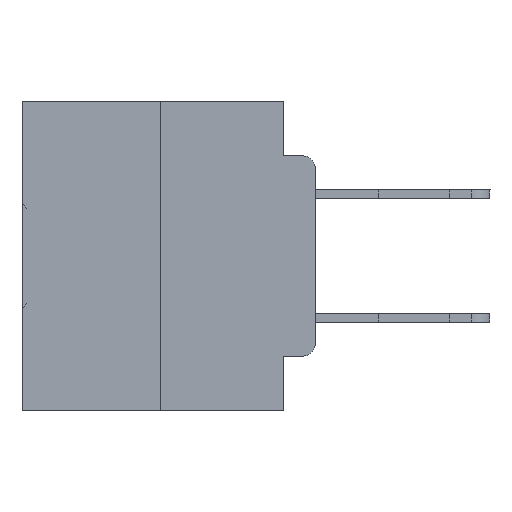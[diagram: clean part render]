
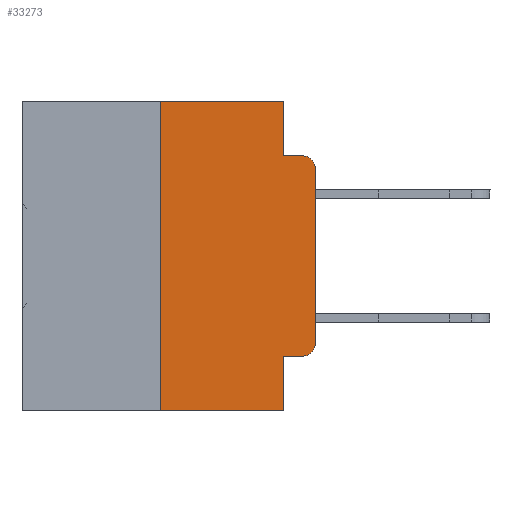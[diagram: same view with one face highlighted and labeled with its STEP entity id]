
A CAD part, left-side view. The second image highlights one B-rep face of the part: STEP entity #33273.
In plain terms, the highlighted planar face has unit normal (-1, 0, 0).
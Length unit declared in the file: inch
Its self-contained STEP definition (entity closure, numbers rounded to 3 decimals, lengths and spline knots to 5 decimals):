
#84 = ORIENTED_EDGE ( 'NONE', *, *, #518, .T. ) ;
#271 = VERTEX_POINT ( 'NONE', #23094 ) ;
#518 = EDGE_CURVE ( 'NONE', #32919, #30354, #25234, .T. ) ;
#638 = CARTESIAN_POINT ( 'NONE',  ( 0., 0.473, -0.5 ) ) ;
#728 = LINE ( 'NONE', #638, #30919 ) ;
#1122 = CARTESIAN_POINT ( 'NONE',  ( 0., 0.051, 0. ) ) ;
#1211 = DIRECTION ( 'NONE',  ( 0., 0., -1. ) ) ;
#1807 = CARTESIAN_POINT ( 'NONE',  ( 0., 0.02, -0.1085 ) ) ;
#1998 = VECTOR ( 'NONE', #28278, 39.37008 ) ;
#2001 = VECTOR ( 'NONE', #23280, 39.37008 ) ;
#2674 = CARTESIAN_POINT ( 'NONE',  ( 0., 0.02, -0.0885 ) ) ;
#3699 = DIRECTION ( 'NONE',  ( 0., -1., 0. ) ) ;
#4699 = CARTESIAN_POINT ( 'NONE',  ( 0., 0.051, -0.0885 ) ) ;
#4810 = CARTESIAN_POINT ( 'NONE',  ( 0., 0.25, 0. ) ) ;
#4901 = FACE_OUTER_BOUND ( 'NONE', #22420, .T. ) ;
#5131 = VERTEX_POINT ( 'NONE', #29912 ) ;
#6466 = LINE ( 'NONE', #28533, #19303 ) ;
#6854 = EDGE_CURVE ( 'NONE', #20907, #25895, #728, .T. ) ;
#7551 = DIRECTION ( 'NONE',  ( -1., 0., 0. ) ) ;
#7661 = ORIENTED_EDGE ( 'NONE', *, *, #16852, .F. ) ;
#8098 = CARTESIAN_POINT ( 'NONE',  ( 0., 0., -0.3915 ) ) ;
#8816 = ORIENTED_EDGE ( 'NONE', *, *, #26133, .T. ) ;
#9095 = CARTESIAN_POINT ( 'NONE',  ( 0., 0.051, -0.4115 ) ) ;
#9280 = ORIENTED_EDGE ( 'NONE', *, *, #27618, .T. ) ;
#10462 = DIRECTION ( 'NONE',  ( 0., 0., -1. ) ) ;
#10625 = ORIENTED_EDGE ( 'NONE', *, *, #31411, .F. ) ;
#11321 = AXIS2_PLACEMENT_3D ( 'NONE', #20862, #7551, #10462 ) ;
#11738 = PLANE ( 'NONE',  #13190 ) ;
#11862 = DIRECTION ( 'NONE',  ( 0., 0., -1. ) ) ;
#12455 = LINE ( 'NONE', #14296, #20310 ) ;
#12686 = DIRECTION ( 'NONE',  ( 0., 0., -1. ) ) ;
#12871 = CARTESIAN_POINT ( 'NONE',  ( 0., 0., -0.1085 ) ) ;
#13122 = CARTESIAN_POINT ( 'NONE',  ( 0., 0.02, -0.4115 ) ) ;
#13190 = AXIS2_PLACEMENT_3D ( 'NONE', #17036, #22673, #1211 ) ;
#14063 = VERTEX_POINT ( 'NONE', #9095 ) ;
#14075 = EDGE_CURVE ( 'NONE', #25152, #5131, #18558, .T. ) ;
#14296 = CARTESIAN_POINT ( 'NONE',  ( 0., 0., 0. ) ) ;
#14378 = LINE ( 'NONE', #1122, #1998 ) ;
#14417 = CARTESIAN_POINT ( 'NONE',  ( 0., 0.473, 0. ) ) ;
#15335 = DIRECTION ( 'NONE',  ( 0., -1., 0. ) ) ;
#15641 = LINE ( 'NONE', #4810, #2001 ) ;
#16852 = EDGE_CURVE ( 'NONE', #20907, #25152, #15641, .T. ) ;
#16993 = ORIENTED_EDGE ( 'NONE', *, *, #14075, .F. ) ;
#17036 = CARTESIAN_POINT ( 'NONE',  ( 0., 0.473, 0. ) ) ;
#17296 = LINE ( 'NONE', #31214, #33454 ) ;
#17738 = AXIS2_PLACEMENT_3D ( 'NONE', #1807, #25504, #11862 ) ;
#18155 = EDGE_CURVE ( 'NONE', #14063, #25895, #6466, .T. ) ;
#18315 = DIRECTION ( 'NONE',  ( 0., -1., 0. ) ) ;
#18558 = LINE ( 'NONE', #14417, #33884 ) ;
#18749 = VERTEX_POINT ( 'NONE', #12871 ) ;
#18763 = CARTESIAN_POINT ( 'NONE',  ( 0., 0.25, 0. ) ) ;
#19303 = VECTOR ( 'NONE', #12686, 39.37008 ) ;
#20310 = VECTOR ( 'NONE', #30365, 39.37008 ) ;
#20862 = CARTESIAN_POINT ( 'NONE',  ( 0., 0.02, -0.3915 ) ) ;
#20907 = VERTEX_POINT ( 'NONE', #31538 ) ;
#22420 = EDGE_LOOP ( 'NONE', ( #8816, #33127, #10625, #22764, #16993, #7661, #24907, #33548, #9280, #84 ) ) ;
#22673 = DIRECTION ( 'NONE',  ( 1., 0., 0. ) ) ;
#22764 = ORIENTED_EDGE ( 'NONE', *, *, #28086, .F. ) ;
#23094 = CARTESIAN_POINT ( 'NONE',  ( 0., 0.051, -0.0885 ) ) ;
#23222 = LINE ( 'NONE', #4699, #32362 ) ;
#23280 = DIRECTION ( 'NONE',  ( 0., 0., 1. ) ) ;
#23941 = VERTEX_POINT ( 'NONE', #2674 ) ;
#24907 = ORIENTED_EDGE ( 'NONE', *, *, #6854, .T. ) ;
#25152 = VERTEX_POINT ( 'NONE', #18763 ) ;
#25234 = CIRCLE ( 'NONE', #11321, 0.02 ) ;
#25504 = DIRECTION ( 'NONE',  ( -1., 0., 0. ) ) ;
#25895 = VERTEX_POINT ( 'NONE', #29121 ) ;
#26133 = EDGE_CURVE ( 'NONE', #30354, #18749, #12455, .T. ) ;
#27618 = EDGE_CURVE ( 'NONE', #14063, #32919, #17296, .T. ) ;
#28086 = EDGE_CURVE ( 'NONE', #5131, #271, #14378, .T. ) ;
#28278 = DIRECTION ( 'NONE',  ( 0., 0., -1. ) ) ;
#28533 = CARTESIAN_POINT ( 'NONE',  ( 0., 0.051, 0. ) ) ;
#29121 = CARTESIAN_POINT ( 'NONE',  ( 0., 0.051, -0.5 ) ) ;
#29461 = EDGE_CURVE ( 'NONE', #18749, #23941, #30853, .T. ) ;
#29912 = CARTESIAN_POINT ( 'NONE',  ( 0., 0.051, 0. ) ) ;
#30354 = VERTEX_POINT ( 'NONE', #8098 ) ;
#30365 = DIRECTION ( 'NONE',  ( 0., 0., 1. ) ) ;
#30853 = CIRCLE ( 'NONE', #17738, 0.02 ) ;
#30919 = VECTOR ( 'NONE', #18315, 39.37008 ) ;
#31063 = DIRECTION ( 'NONE',  ( 0., -1., 0. ) ) ;
#31214 = CARTESIAN_POINT ( 'NONE',  ( 0., 0.051, -0.4115 ) ) ;
#31411 = EDGE_CURVE ( 'NONE', #271, #23941, #23222, .T. ) ;
#31538 = CARTESIAN_POINT ( 'NONE',  ( 0., 0.25, -0.5 ) ) ;
#32362 = VECTOR ( 'NONE', #31063, 39.37008 ) ;
#32919 = VERTEX_POINT ( 'NONE', #13122 ) ;
#33127 = ORIENTED_EDGE ( 'NONE', *, *, #29461, .T. ) ;
#33273 = ADVANCED_FACE ( 'NONE', ( #4901 ), #11738, .F. ) ;
#33454 = VECTOR ( 'NONE', #15335, 39.37008 ) ;
#33548 = ORIENTED_EDGE ( 'NONE', *, *, #18155, .F. ) ;
#33884 = VECTOR ( 'NONE', #3699, 39.37008 ) ;
